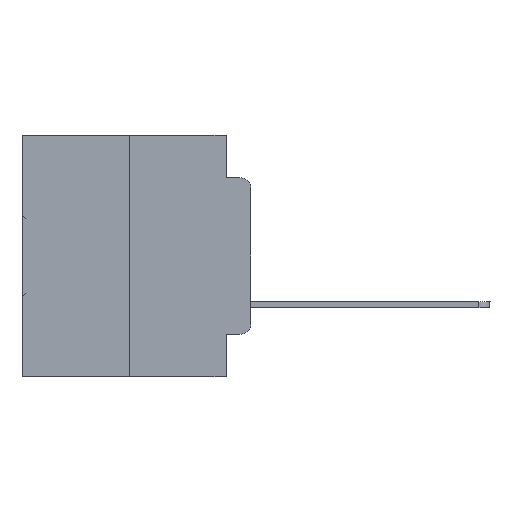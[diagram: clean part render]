
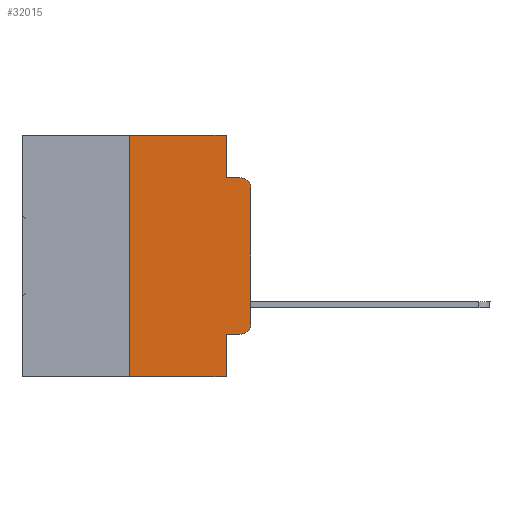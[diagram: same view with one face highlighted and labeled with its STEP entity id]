
A CAD part, left-side view. The second image highlights one B-rep face of the part: STEP entity #32015.
In plain terms, the highlighted planar face has unit normal (-1, 0, 0).
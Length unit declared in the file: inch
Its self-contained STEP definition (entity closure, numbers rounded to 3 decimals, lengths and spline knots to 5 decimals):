
#167 = CARTESIAN_POINT ( 'NONE',  ( 0., 0.051, -0.5 ) ) ;
#626 = EDGE_CURVE ( 'NONE', #32494, #17168, #10502, .T. ) ;
#844 = CIRCLE ( 'NONE', #4333, 0.02 ) ;
#1139 = ORIENTED_EDGE ( 'NONE', *, *, #26011, .F. ) ;
#1182 = VERTEX_POINT ( 'NONE', #167 ) ;
#1392 = FACE_OUTER_BOUND ( 'NONE', #15479, .T. ) ;
#1534 = CARTESIAN_POINT ( 'NONE',  ( 0., 0.051, 0. ) ) ;
#1570 = VECTOR ( 'NONE', #6739, 39.37008 ) ;
#2306 = VECTOR ( 'NONE', #21938, 39.37008 ) ;
#3018 = AXIS2_PLACEMENT_3D ( 'NONE', #32889, #21919, #21803 ) ;
#3134 = DIRECTION ( 'NONE',  ( 1., 0., 0. ) ) ;
#3280 = CARTESIAN_POINT ( 'NONE',  ( 0., 0.051, -0.4115 ) ) ;
#3305 = DIRECTION ( 'NONE',  ( 0., -1., 0. ) ) ;
#3487 = LINE ( 'NONE', #20400, #9935 ) ;
#4333 = AXIS2_PLACEMENT_3D ( 'NONE', #27914, #6482, #18005 ) ;
#4767 = CARTESIAN_POINT ( 'NONE',  ( 0., 0.02, -0.0885 ) ) ;
#4898 = VERTEX_POINT ( 'NONE', #21261 ) ;
#5348 = CARTESIAN_POINT ( 'NONE',  ( 0., 0., 0. ) ) ;
#5573 = ORIENTED_EDGE ( 'NONE', *, *, #20297, .F. ) ;
#6482 = DIRECTION ( 'NONE',  ( -1., 0., 0. ) ) ;
#6739 = DIRECTION ( 'NONE',  ( 0., -1., 0. ) ) ;
#6962 = CARTESIAN_POINT ( 'NONE',  ( 0., 0.051, -0.0885 ) ) ;
#7436 = VECTOR ( 'NONE', #24083, 39.37008 ) ;
#8005 = CARTESIAN_POINT ( 'NONE',  ( 0., 0.051, -0.0885 ) ) ;
#8298 = LINE ( 'NONE', #27009, #7436 ) ;
#8717 = EDGE_CURVE ( 'NONE', #4898, #1182, #3487, .T. ) ;
#9935 = VECTOR ( 'NONE', #17158, 39.37008 ) ;
#10502 = LINE ( 'NONE', #5348, #2306 ) ;
#11905 = CARTESIAN_POINT ( 'NONE',  ( 0., 0.473, 0. ) ) ;
#12038 = ORIENTED_EDGE ( 'NONE', *, *, #24716, .F. ) ;
#12218 = DIRECTION ( 'NONE',  ( 0., 0., 1. ) ) ;
#12293 = LINE ( 'NONE', #6962, #20869 ) ;
#12478 = DIRECTION ( 'NONE',  ( 0., -1., 0. ) ) ;
#12580 = VERTEX_POINT ( 'NONE', #4767 ) ;
#13694 = CARTESIAN_POINT ( 'NONE',  ( 0., 0., -0.3915 ) ) ;
#15479 = EDGE_LOOP ( 'NONE', ( #32376, #34108, #28435, #12038, #1139, #5573, #28860, #35017, #21291, #24010 ) ) ;
#15886 = CIRCLE ( 'NONE', #3018, 0.02 ) ;
#16233 = LINE ( 'NONE', #11905, #1570 ) ;
#16746 = CARTESIAN_POINT ( 'NONE',  ( 0., 0., -0.1085 ) ) ;
#16987 = CARTESIAN_POINT ( 'NONE',  ( 0., 0.25, 0. ) ) ;
#17158 = DIRECTION ( 'NONE',  ( 0., -1., 0. ) ) ;
#17168 = VERTEX_POINT ( 'NONE', #16746 ) ;
#17937 = EDGE_CURVE ( 'NONE', #26786, #12580, #12293, .T. ) ;
#18005 = DIRECTION ( 'NONE',  ( 0., 0., -1. ) ) ;
#18285 = EDGE_CURVE ( 'NONE', #33957, #32494, #844, .T. ) ;
#19403 = CARTESIAN_POINT ( 'NONE',  ( 0., 0.473, 0. ) ) ;
#19641 = DIRECTION ( 'NONE',  ( 0., 0., -1. ) ) ;
#19715 = VECTOR ( 'NONE', #32137, 39.37008 ) ;
#20297 = EDGE_CURVE ( 'NONE', #4898, #30765, #29767, .T. ) ;
#20400 = CARTESIAN_POINT ( 'NONE',  ( 0., 0.473, -0.5 ) ) ;
#20511 = CARTESIAN_POINT ( 'NONE',  ( 0., 0.25, 0. ) ) ;
#20869 = VECTOR ( 'NONE', #12478, 39.37008 ) ;
#21261 = CARTESIAN_POINT ( 'NONE',  ( 0., 0.25, -0.5 ) ) ;
#21291 = ORIENTED_EDGE ( 'NONE', *, *, #22065, .T. ) ;
#21803 = DIRECTION ( 'NONE',  ( 0., 0., -1. ) ) ;
#21919 = DIRECTION ( 'NONE',  ( -1., 0., 0. ) ) ;
#21938 = DIRECTION ( 'NONE',  ( 0., 0., 1. ) ) ;
#22065 = EDGE_CURVE ( 'NONE', #22653, #33957, #34366, .T. ) ;
#22430 = VECTOR ( 'NONE', #12218, 39.37008 ) ;
#22653 = VERTEX_POINT ( 'NONE', #3280 ) ;
#23471 = CARTESIAN_POINT ( 'NONE',  ( 0., 0.02, -0.4115 ) ) ;
#24010 = ORIENTED_EDGE ( 'NONE', *, *, #18285, .T. ) ;
#24083 = DIRECTION ( 'NONE',  ( 0., 0., -1. ) ) ;
#24716 = EDGE_CURVE ( 'NONE', #31367, #26786, #31794, .T. ) ;
#25164 = PLANE ( 'NONE',  #31206 ) ;
#26011 = EDGE_CURVE ( 'NONE', #30765, #31367, #16233, .T. ) ;
#26786 = VERTEX_POINT ( 'NONE', #8005 ) ;
#27009 = CARTESIAN_POINT ( 'NONE',  ( 0., 0.051, 0. ) ) ;
#27914 = CARTESIAN_POINT ( 'NONE',  ( 0., 0.02, -0.3915 ) ) ;
#28435 = ORIENTED_EDGE ( 'NONE', *, *, #17937, .F. ) ;
#28860 = ORIENTED_EDGE ( 'NONE', *, *, #8717, .T. ) ;
#29767 = LINE ( 'NONE', #20511, #22430 ) ;
#30663 = EDGE_CURVE ( 'NONE', #17168, #12580, #15886, .T. ) ;
#30765 = VERTEX_POINT ( 'NONE', #16987 ) ;
#31206 = AXIS2_PLACEMENT_3D ( 'NONE', #19403, #3134, #19641 ) ;
#31367 = VERTEX_POINT ( 'NONE', #33808 ) ;
#31794 = LINE ( 'NONE', #1534, #19715 ) ;
#31912 = EDGE_CURVE ( 'NONE', #22653, #1182, #8298, .T. ) ;
#32015 = ADVANCED_FACE ( 'NONE', ( #1392 ), #25164, .F. ) ;
#32137 = DIRECTION ( 'NONE',  ( 0., 0., -1. ) ) ;
#32376 = ORIENTED_EDGE ( 'NONE', *, *, #626, .T. ) ;
#32494 = VERTEX_POINT ( 'NONE', #13694 ) ;
#32889 = CARTESIAN_POINT ( 'NONE',  ( 0., 0.02, -0.1085 ) ) ;
#33767 = CARTESIAN_POINT ( 'NONE',  ( 0., 0.051, -0.4115 ) ) ;
#33808 = CARTESIAN_POINT ( 'NONE',  ( 0., 0.051, 0. ) ) ;
#33944 = VECTOR ( 'NONE', #3305, 39.37008 ) ;
#33957 = VERTEX_POINT ( 'NONE', #23471 ) ;
#34108 = ORIENTED_EDGE ( 'NONE', *, *, #30663, .T. ) ;
#34366 = LINE ( 'NONE', #33767, #33944 ) ;
#35017 = ORIENTED_EDGE ( 'NONE', *, *, #31912, .F. ) ;
